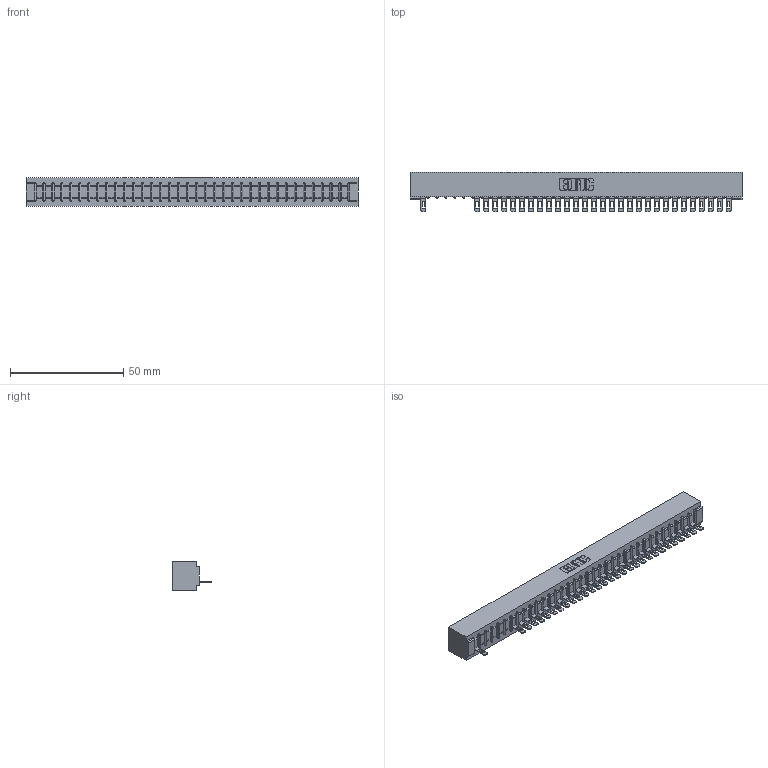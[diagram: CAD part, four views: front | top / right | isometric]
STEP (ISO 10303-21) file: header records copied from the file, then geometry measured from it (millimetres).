
FILE_DESCRIPTION (( 'STEP AP203' ), '1' );
FILE_NAME ('357-035-501-101.STEP', '2018-08-10T04:20:24', ( '' ), ( '' ), 'SwSTEP 2.0', 'SolidWorks 2016', '' );
FILE_SCHEMA (( 'CONFIG_CONTROL_DESIGN' ));
Length unit declared in the file: inch
Products named in the file (3): 357-035-501-101; 307 Part_No Mounting Lugs; 307-290-002_501
Assembly tree (31 placements, depth 2):
  357-035-501-101
    307 Part_No Mounting Lugs
    307-290-002_501  x30
Bounding box: 146.56 x 17.42 x 12.7 mm (x, y, z)
Volume: 16070.6 mm3; surface area: 19678.7 mm2
Topology: 31 solids, 31 shells, 2526 faces, 7759 edges, 5074 vertices
Faces by surface type: plane 1446, cylinder 1008, sphere 72
Entity records: 31224 total; most frequent: CARTESIAN_POINT 5287, ORIENTED_EDGE 5282, DIRECTION 5137, EDGE_CURVE 2641, LINE 2017, VECTOR 2017, VERTEX_POINT 1710, AXIS2_PLACEMENT_3D 1560
